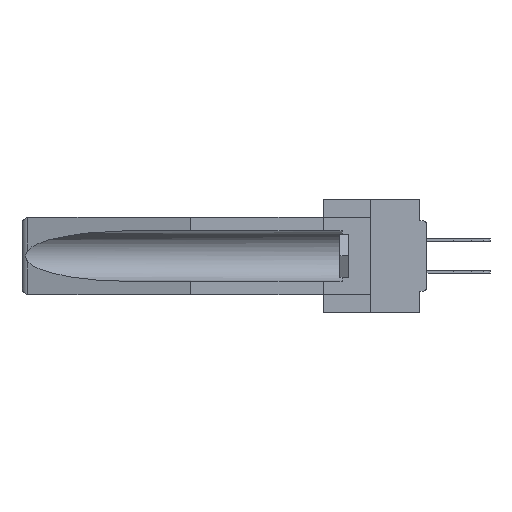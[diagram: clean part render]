
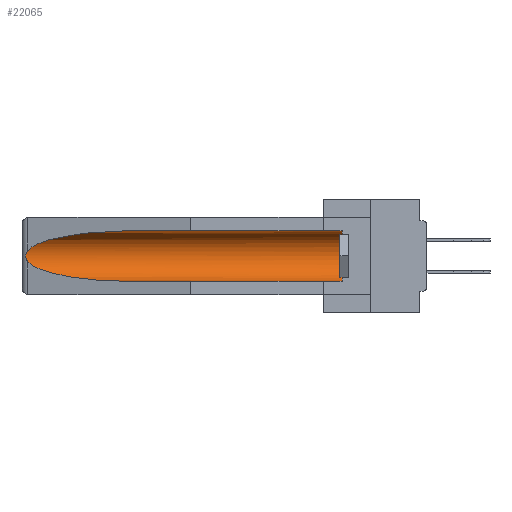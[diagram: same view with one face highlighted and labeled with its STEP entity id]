
A CAD part, left-side view. The second image highlights one B-rep face of the part: STEP entity #22065.
In plain terms, the highlighted cylindrical face has radius 2.857 mm (diameter 5.715 mm), a partial arc.
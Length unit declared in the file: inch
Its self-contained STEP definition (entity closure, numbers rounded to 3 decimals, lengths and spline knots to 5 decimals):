
#206 = CIRCLE ( 'NONE', #42616, 0.1125 ) ;
#503 = DIRECTION ( 'NONE',  ( 0., 1., 0. ) ) ;
#1819 = VERTEX_POINT ( 'NONE', #34471 ) ;
#2545 = EDGE_CURVE ( 'NONE', #21429, #6709, #44080, .T. ) ;
#6288 = EDGE_CURVE ( 'NONE', #1819, #28167, #12753, .T. ) ;
#6619 = CARTESIAN_POINT ( 'NONE',  ( 0.26655, 1.53094, -0.18657 ) ) ;
#6709 = VERTEX_POINT ( 'NONE', #27396 ) ;
#7300 = EDGE_CURVE ( 'NONE', #38307, #26155, #13745, .T. ) ;
#9662 = CARTESIAN_POINT ( 'NONE',  ( 0.26537, 1.52718, -0.14972 ) ) ;
#9710 = CARTESIAN_POINT ( 'NONE',  ( 0.26537, 1.52718, -0.19328 ) ) ;
#9998 = VECTOR ( 'NONE', #23767, 39.37008 ) ;
#10703 = CARTESIAN_POINT ( 'NONE',  ( 0.21114, 1.30732, -0.059 ) ) ;
#11874 = DIRECTION ( 'NONE',  ( 0., 1., 0. ) ) ;
#12753 = B_SPLINE_CURVE_WITH_KNOTS ( 'NONE', 3,
 ( #9662, #30754, #20042, #17184, #16893, #41079, #27540, #6619, #41501, #37864 ),
 .UNSPECIFIED., .F., .F.,
 ( 4, 2, 2, 2, 4 ),
 ( 0., 0.00029, 0.00058, 0.00087, 0.00117 ),
 .UNSPECIFIED. ) ;
#13420 = CARTESIAN_POINT ( 'NONE',  ( 0.155, 0.126, -0.1715 ) ) ;
#13745 = LINE ( 'NONE', #23626, #9998 ) ;
#16893 = CARTESIAN_POINT ( 'NONE',  ( 0.2675, 1.53308, -0.16763 ) ) ;
#17184 = CARTESIAN_POINT ( 'NONE',  ( 0.2673, 1.5327, -0.16383 ) ) ;
#17881 = CARTESIAN_POINT ( 'NONE',  ( 0.155, 0.126, -0.059 ) ) ;
#20042 = CARTESIAN_POINT ( 'NONE',  ( 0.26654, 1.53092, -0.15636 ) ) ;
#20684 = EDGE_CURVE ( 'NONE', #21429, #38307, #206, .T. ) ;
#20762 = AXIS2_PLACEMENT_3D ( 'NONE', #29322, #11874, #32989 ) ;
#21027 = ORIENTED_EDGE ( 'NONE', *, *, #39856, .T. ) ;
#21429 = VERTEX_POINT ( 'NONE', #41337 ) ;
#22065 = ADVANCED_FACE ( 'NONE', ( #29701 ), #42729, .F. ) ;
#23626 = CARTESIAN_POINT ( 'NONE',  ( 0.155, -0.30754, -0.059 ) ) ;
#23767 = DIRECTION ( 'NONE',  ( 0., 1., 0. ) ) ;
#23856 = DIRECTION ( 'NONE',  ( 0., 0., 1. ) ) ;
#23909 = CARTESIAN_POINT ( 'NONE',  ( 0.155, 1.07973, -0.284 ) ) ;
#26155 = VERTEX_POINT ( 'NONE', #36501 ) ;
#26355 = ORIENTED_EDGE ( 'NONE', *, *, #35243, .T. ) ;
#27396 = CARTESIAN_POINT ( 'NONE',  ( 0.155, 1.07973, -0.284 ) ) ;
#27540 = CARTESIAN_POINT ( 'NONE',  ( 0.2673, 1.53269, -0.17917 ) ) ;
#27886 = ORIENTED_EDGE ( 'NONE', *, *, #6288, .T. ) ;
#28167 = VERTEX_POINT ( 'NONE', #39537 ) ;
#29322 = CARTESIAN_POINT ( 'NONE',  ( 0.155, -0.30754, -0.1715 ) ) ;
#29701 = FACE_OUTER_BOUND ( 'NONE', #33277, .T. ) ;
#30754 = CARTESIAN_POINT ( 'NONE',  ( 0.26597, 1.52961, -0.15275 ) ) ;
#30927 = CARTESIAN_POINT ( 'NONE',  ( 0.155, -0.30754, -0.284 ) ) ;
#31599 = CARTESIAN_POINT ( 'NONE',  ( 0.155, 1.07973, -0.059 ) ) ;
#32587 = ORIENTED_EDGE ( 'NONE', *, *, #20684, .T. ) ;
#32650 = VECTOR ( 'NONE', #503, 39.37008 ) ;
#32989 = DIRECTION ( 'NONE',  ( 0., 0., 1. ) ) ;
#33277 = EDGE_LOOP ( 'NONE', ( #21027, #27886, #26355, #40793, #32587, #42421 ) ) ;
#33288 = CARTESIAN_POINT ( 'NONE',  ( 0.25451, 1.48313, -0.09465 ) ) ;
#33708 = CARTESIAN_POINT ( 'NONE',  ( 0.25451, 1.48313, -0.24835 ) ) ;
#34471 = CARTESIAN_POINT ( 'NONE',  ( 0.26537, 1.52718, -0.14972 ) ) ;
#35243 = EDGE_CURVE ( 'NONE', #28167, #6709, #44742, .T. ) ;
#36501 = CARTESIAN_POINT ( 'NONE',  ( 0.155, 1.07973, -0.059 ) ) ;
#36822 = CARTESIAN_POINT ( 'NONE',  ( 0.26537, 1.52718, -0.14972 ) ) ;
#37616 = CARTESIAN_POINT ( 'NONE',  ( 0.21114, 1.30732, -0.284 ) ) ;
#37864 = CARTESIAN_POINT ( 'NONE',  ( 0.26537, 1.52718, -0.19328 ) ) ;
#38307 = VERTEX_POINT ( 'NONE', #17881 ) ;
#39537 = CARTESIAN_POINT ( 'NONE',  ( 0.26537, 1.52718, -0.19328 ) ) ;
#39856 = EDGE_CURVE ( 'NONE', #26155, #1819, #42805, .T. ) ;
#40793 = ORIENTED_EDGE ( 'NONE', *, *, #2545, .F. ) ;
#41079 = CARTESIAN_POINT ( 'NONE',  ( 0.2675, 1.53308, -0.17534 ) ) ;
#41206 = DIRECTION ( 'NONE',  ( 0., -1., 0. ) ) ;
#41337 = CARTESIAN_POINT ( 'NONE',  ( 0.155, 0.126, -0.284 ) ) ;
#41501 = CARTESIAN_POINT ( 'NONE',  ( 0.26597, 1.5296, -0.19026 ) ) ;
#42421 = ORIENTED_EDGE ( 'NONE', *, *, #7300, .T. ) ;
#42616 = AXIS2_PLACEMENT_3D ( 'NONE', #13420, #41206, #23856 ) ;
#42729 = CYLINDRICAL_SURFACE ( 'NONE', #20762, 0.1125 ) ;
#42805 =( BOUNDED_CURVE ( )  B_SPLINE_CURVE ( 3, ( #31599, #10703, #33288, #36822 ),
 .UNSPECIFIED., .F., .F. ) 
 B_SPLINE_CURVE_WITH_KNOTS ( ( 4, 4 ),
 ( 4.71239, 6.08839 ),
 .UNSPECIFIED. ) 
 CURVE ( )  GEOMETRIC_REPRESENTATION_ITEM ( )  RATIONAL_B_SPLINE_CURVE ( ( 1., 0.848, 0.848, 1. ) ) 
 REPRESENTATION_ITEM ( '' )  );
#44080 = LINE ( 'NONE', #30927, #32650 ) ;
#44742 =( BOUNDED_CURVE ( )  B_SPLINE_CURVE ( 3, ( #9710, #33708, #37616, #23909 ),
 .UNSPECIFIED., .F., .T. ) 
 B_SPLINE_CURVE_WITH_KNOTS ( ( 4, 4 ),
 ( 0.1948, 1.5708 ),
 .UNSPECIFIED. ) 
 CURVE ( )  GEOMETRIC_REPRESENTATION_ITEM ( )  RATIONAL_B_SPLINE_CURVE ( ( 1., 0.848, 0.848, 1. ) ) 
 REPRESENTATION_ITEM ( '' )  );
